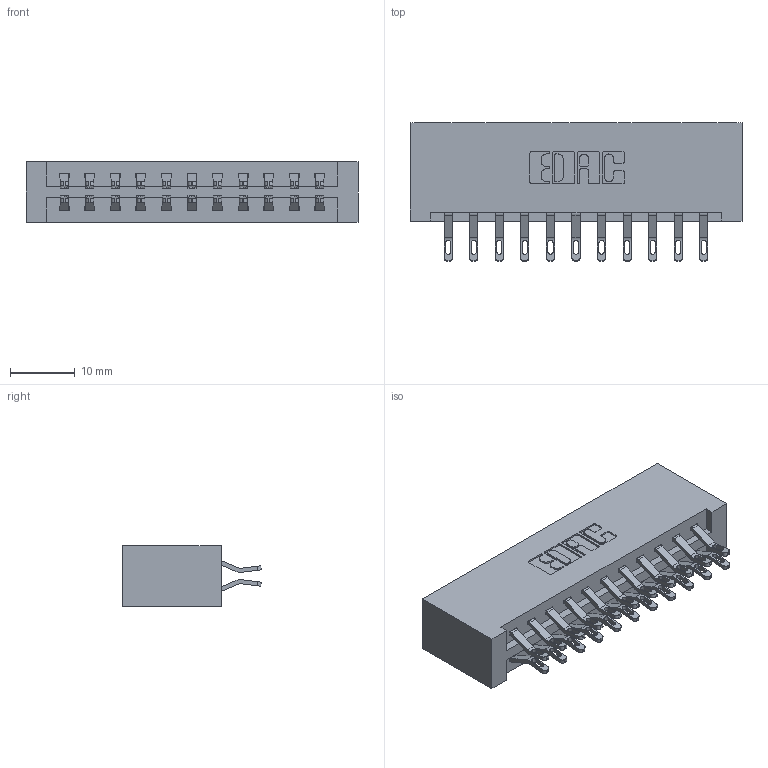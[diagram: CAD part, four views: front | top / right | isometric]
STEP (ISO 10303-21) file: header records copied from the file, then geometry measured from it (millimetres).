
FILE_DESCRIPTION (( 'STEP AP203' ), '1' );
FILE_NAME ('387-022-555-201.STEP', '2019-10-16T17:05:10', ( '' ), ( '' ), 'SwSTEP 2.0', 'SolidWorks 2016', '' );
FILE_SCHEMA (( 'CONFIG_CONTROL_DESIGN' ));
Length unit declared in the file: inch
Products named in the file (3): 387-022-555-201; 345-292-001_555 Tail; 337 Part_No Mounting Lugs
Assembly tree (23 placements, depth 2):
  387-022-555-201
    337 Part_No Mounting Lugs
    345-292-001_555 Tail  x22
Bounding box: 51.46 x 21.47 x 9.4 mm (x, y, z)
Volume: 5835.2 mm3; surface area: 6592.2 mm2
Topology: 23 solids, 23 shells, 1426 faces, 4445 edges, 2962 vertices
Faces by surface type: plane 858, cylinder 568
Entity records: 12587 total; most frequent: CARTESIAN_POINT 2180, ORIENTED_EDGE 2086, DIRECTION 1875, EDGE_CURVE 1043, VECTOR 903, LINE 903, VERTEX_POINT 694, AXIS2_PLACEMENT_3D 486
